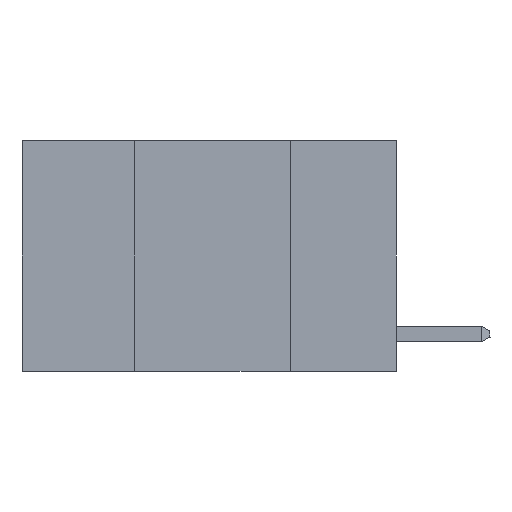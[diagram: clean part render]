
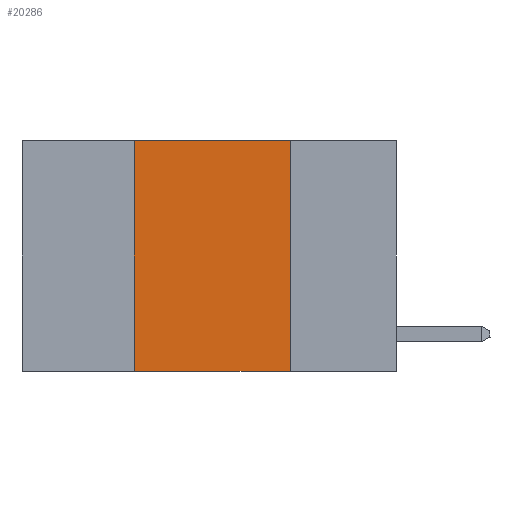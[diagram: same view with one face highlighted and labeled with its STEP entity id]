
A CAD part, left-side view. The second image highlights one B-rep face of the part: STEP entity #20286.
In plain terms, the highlighted planar face has unit normal (-1, 0, 0).
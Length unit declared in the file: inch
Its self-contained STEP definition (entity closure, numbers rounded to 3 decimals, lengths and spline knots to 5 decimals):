
#679 = CARTESIAN_POINT ( 'NONE',  ( 0., 0.42, 0. ) ) ;
#1220 = ORIENTED_EDGE ( 'NONE', *, *, #17502, .T. ) ;
#2469 = ORIENTED_EDGE ( 'NONE', *, *, #13326, .F. ) ;
#2746 = LINE ( 'NONE', #7938, #17920 ) ;
#3494 = CARTESIAN_POINT ( 'NONE',  ( 0., 0.42, -0.37 ) ) ;
#4943 = DIRECTION ( 'NONE',  ( 0., -1., 0. ) ) ;
#5296 = FACE_OUTER_BOUND ( 'NONE', #15368, .T. ) ;
#6236 = CARTESIAN_POINT ( 'NONE',  ( 0., 0.17, 0. ) ) ;
#6653 = AXIS2_PLACEMENT_3D ( 'NONE', #11450, #19211, #13275 ) ;
#7938 = CARTESIAN_POINT ( 'NONE',  ( 0., 0.6, -0.37 ) ) ;
#8474 = CARTESIAN_POINT ( 'NONE',  ( 0., 0.6, 0. ) ) ;
#8758 = LINE ( 'NONE', #679, #19045 ) ;
#11450 = CARTESIAN_POINT ( 'NONE',  ( 0., 0.6, 0. ) ) ;
#11750 = ORIENTED_EDGE ( 'NONE', *, *, #14629, .F. ) ;
#12121 = CARTESIAN_POINT ( 'NONE',  ( 0., 0.42, 0. ) ) ;
#13275 = DIRECTION ( 'NONE',  ( 0., 0., -1. ) ) ;
#13326 = EDGE_CURVE ( 'NONE', #18690, #21599, #22740, .T. ) ;
#13790 = CARTESIAN_POINT ( 'NONE',  ( 0., 0.17, -0.37 ) ) ;
#14629 = EDGE_CURVE ( 'NONE', #24807, #18690, #8758, .T. ) ;
#15368 = EDGE_LOOP ( 'NONE', ( #18400, #2469, #11750, #1220 ) ) ;
#15725 = DIRECTION ( 'NONE',  ( 0., 0., -1. ) ) ;
#15846 = DIRECTION ( 'NONE',  ( 0., -1., 0. ) ) ;
#17502 = EDGE_CURVE ( 'NONE', #24807, #20407, #2746, .T. ) ;
#17545 = LINE ( 'NONE', #6236, #21660 ) ;
#17920 = VECTOR ( 'NONE', #15846, 39.37008 ) ;
#18341 = DIRECTION ( 'NONE',  ( 0., 0., 1. ) ) ;
#18400 = ORIENTED_EDGE ( 'NONE', *, *, #18760, .F. ) ;
#18690 = VERTEX_POINT ( 'NONE', #12121 ) ;
#18760 = EDGE_CURVE ( 'NONE', #21599, #20407, #17545, .T. ) ;
#19045 = VECTOR ( 'NONE', #18341, 39.37008 ) ;
#19183 = CARTESIAN_POINT ( 'NONE',  ( 0., 0.17, 0. ) ) ;
#19211 = DIRECTION ( 'NONE',  ( 1., 0., 0. ) ) ;
#20286 = ADVANCED_FACE ( 'NONE', ( #5296 ), #22992, .F. ) ;
#20407 = VERTEX_POINT ( 'NONE', #13790 ) ;
#21599 = VERTEX_POINT ( 'NONE', #19183 ) ;
#21660 = VECTOR ( 'NONE', #15725, 39.37008 ) ;
#22740 = LINE ( 'NONE', #8474, #24661 ) ;
#22992 = PLANE ( 'NONE',  #6653 ) ;
#24661 = VECTOR ( 'NONE', #4943, 39.37008 ) ;
#24807 = VERTEX_POINT ( 'NONE', #3494 ) ;
